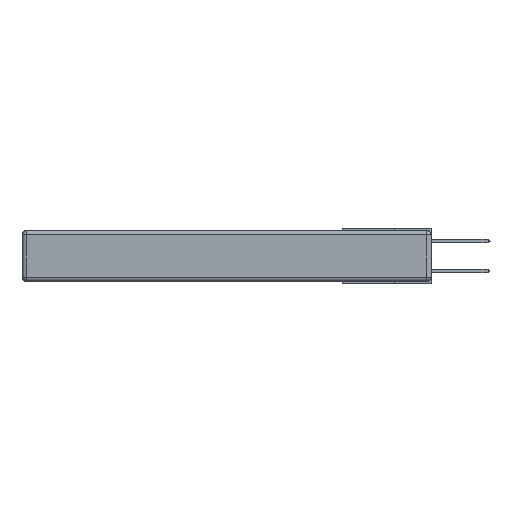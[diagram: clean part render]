
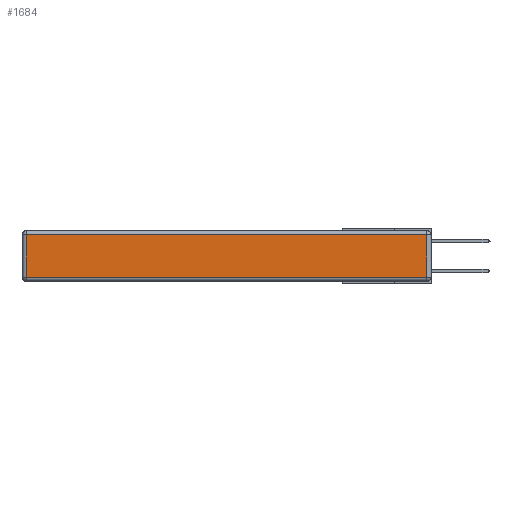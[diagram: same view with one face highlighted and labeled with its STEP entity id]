
A CAD part, left-side view. The second image highlights one B-rep face of the part: STEP entity #1684.
In plain terms, the highlighted planar face has unit normal (-1, 0, 0).
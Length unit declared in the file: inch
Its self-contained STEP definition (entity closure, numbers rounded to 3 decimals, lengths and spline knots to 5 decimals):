
#1684 = ADVANCED_FACE ( 'NONE', ( #20250 ), #13300, .T. ) ;
#4101 = CARTESIAN_POINT ( 'NONE',  ( 0., 0.03, -0.343 ) ) ;
#5707 = CARTESIAN_POINT ( 'NONE',  ( 0., 2.75, -0.03 ) ) ;
#7053 = LINE ( 'NONE', #14773, #12990 ) ;
#7928 = EDGE_CURVE ( 'NONE', #10687, #13040, #32414, .T. ) ;
#7965 = DIRECTION ( 'NONE',  ( 0., 0., 1. ) ) ;
#8849 = EDGE_CURVE ( 'NONE', #14480, #20050, #27718, .T. ) ;
#9530 = DIRECTION ( 'NONE',  ( 0., -1., 0. ) ) ;
#10323 = VECTOR ( 'NONE', #14131, 39.37008 ) ;
#10687 = VERTEX_POINT ( 'NONE', #30278 ) ;
#11319 = EDGE_CURVE ( 'NONE', #13040, #14480, #32109, .T. ) ;
#12135 = CARTESIAN_POINT ( 'NONE',  ( 0., 2.72, -0.343 ) ) ;
#12990 = VECTOR ( 'NONE', #9530, 39.37008 ) ;
#13040 = VERTEX_POINT ( 'NONE', #24822 ) ;
#13300 = PLANE ( 'NONE',  #21019 ) ;
#14022 = EDGE_LOOP ( 'NONE', ( #24270, #24971, #20501, #17664 ) ) ;
#14131 = DIRECTION ( 'NONE',  ( 0., 1., 0. ) ) ;
#14480 = VERTEX_POINT ( 'NONE', #14785 ) ;
#14773 = CARTESIAN_POINT ( 'NONE',  ( 0., 0., -0.313 ) ) ;
#14785 = CARTESIAN_POINT ( 'NONE',  ( 0., 2.72, -0.03 ) ) ;
#16003 = DIRECTION ( 'NONE',  ( 0., 0., 1. ) ) ;
#17664 = ORIENTED_EDGE ( 'NONE', *, *, #8849, .T. ) ;
#20050 = VERTEX_POINT ( 'NONE', #29624 ) ;
#20250 = FACE_OUTER_BOUND ( 'NONE', #14022, .T. ) ;
#20501 = ORIENTED_EDGE ( 'NONE', *, *, #11319, .T. ) ;
#21019 = AXIS2_PLACEMENT_3D ( 'NONE', #26307, #21292, #7965 ) ;
#21292 = DIRECTION ( 'NONE',  ( -1., 0., 0. ) ) ;
#23258 = EDGE_CURVE ( 'NONE', #20050, #10687, #7053, .T. ) ;
#24270 = ORIENTED_EDGE ( 'NONE', *, *, #23258, .T. ) ;
#24822 = CARTESIAN_POINT ( 'NONE',  ( 0., 0.03, -0.03 ) ) ;
#24971 = ORIENTED_EDGE ( 'NONE', *, *, #7928, .T. ) ;
#25223 = VECTOR ( 'NONE', #31129, 39.37008 ) ;
#26307 = CARTESIAN_POINT ( 'NONE',  ( 0., 0., -0.343 ) ) ;
#27718 = LINE ( 'NONE', #12135, #25223 ) ;
#29624 = CARTESIAN_POINT ( 'NONE',  ( 0., 2.72, -0.313 ) ) ;
#30278 = CARTESIAN_POINT ( 'NONE',  ( 0., 0.03, -0.313 ) ) ;
#31118 = VECTOR ( 'NONE', #16003, 39.37008 ) ;
#31129 = DIRECTION ( 'NONE',  ( 0., 0., -1. ) ) ;
#32109 = LINE ( 'NONE', #5707, #10323 ) ;
#32414 = LINE ( 'NONE', #4101, #31118 ) ;
